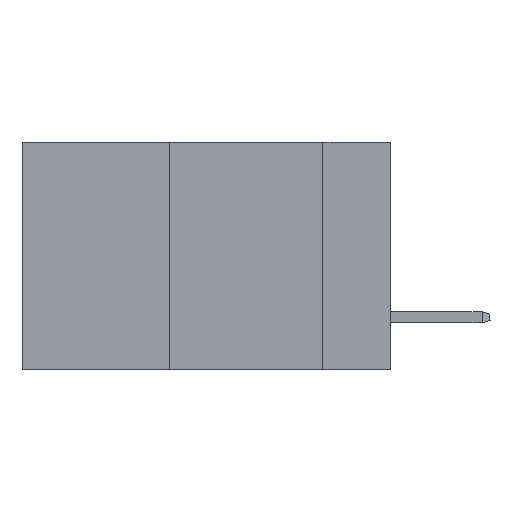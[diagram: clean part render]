
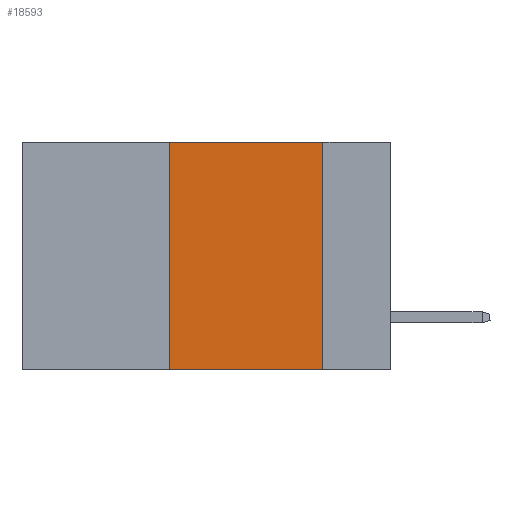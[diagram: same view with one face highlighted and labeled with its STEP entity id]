
A CAD part, left-side view. The second image highlights one B-rep face of the part: STEP entity #18593.
In plain terms, the highlighted planar face has unit normal (-1, 0, 0).
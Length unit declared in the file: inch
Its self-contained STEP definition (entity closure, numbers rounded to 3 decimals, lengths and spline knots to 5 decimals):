
#859 = CARTESIAN_POINT ( 'NONE',  ( 0., 0.11, -0.37 ) ) ;
#862 = CARTESIAN_POINT ( 'NONE',  ( 0., 0.36, 0. ) ) ;
#1056 = DIRECTION ( 'NONE',  ( 0., 0., 1. ) ) ;
#1254 = DIRECTION ( 'NONE',  ( 0., 0., -1. ) ) ;
#1319 = DIRECTION ( 'NONE',  ( 1., 0., 0. ) ) ;
#1737 = VECTOR ( 'NONE', #16440, 39.37008 ) ;
#1964 = ORIENTED_EDGE ( 'NONE', *, *, #2080, .F. ) ;
#2080 = EDGE_CURVE ( 'NONE', #9829, #5342, #14048, .T. ) ;
#2199 = CARTESIAN_POINT ( 'NONE',  ( 0., 0.36, -0.37 ) ) ;
#2877 = PLANE ( 'NONE',  #5099 ) ;
#3153 = VERTEX_POINT ( 'NONE', #859 ) ;
#3887 = LINE ( 'NONE', #7358, #1737 ) ;
#4326 = VERTEX_POINT ( 'NONE', #2199 ) ;
#4347 = CARTESIAN_POINT ( 'NONE',  ( 0., 0.11, 0. ) ) ;
#5099 = AXIS2_PLACEMENT_3D ( 'NONE', #8757, #1319, #1254 ) ;
#5342 = VERTEX_POINT ( 'NONE', #4347 ) ;
#5566 = EDGE_LOOP ( 'NONE', ( #11028, #1964, #9701, #9909 ) ) ;
#6669 = VECTOR ( 'NONE', #1056, 39.37008 ) ;
#7358 = CARTESIAN_POINT ( 'NONE',  ( 0., 0.6, -0.37 ) ) ;
#7507 = FACE_OUTER_BOUND ( 'NONE', #5566, .T. ) ;
#7860 = EDGE_CURVE ( 'NONE', #4326, #9829, #15578, .T. ) ;
#8757 = CARTESIAN_POINT ( 'NONE',  ( 0., 0.6, 0. ) ) ;
#8834 = VECTOR ( 'NONE', #13180, 39.37008 ) ;
#9701 = ORIENTED_EDGE ( 'NONE', *, *, #7860, .F. ) ;
#9829 = VERTEX_POINT ( 'NONE', #15761 ) ;
#9909 = ORIENTED_EDGE ( 'NONE', *, *, #16830, .T. ) ;
#10369 = DIRECTION ( 'NONE',  ( 0., 0., -1. ) ) ;
#11028 = ORIENTED_EDGE ( 'NONE', *, *, #11609, .F. ) ;
#11609 = EDGE_CURVE ( 'NONE', #5342, #3153, #17215, .T. ) ;
#13180 = DIRECTION ( 'NONE',  ( 0., -1., 0. ) ) ;
#14048 = LINE ( 'NONE', #19174, #8834 ) ;
#15578 = LINE ( 'NONE', #862, #6669 ) ;
#15761 = CARTESIAN_POINT ( 'NONE',  ( 0., 0.36, 0. ) ) ;
#16440 = DIRECTION ( 'NONE',  ( 0., -1., 0. ) ) ;
#16830 = EDGE_CURVE ( 'NONE', #4326, #3153, #3887, .T. ) ;
#17215 = LINE ( 'NONE', #19208, #19325 ) ;
#18593 = ADVANCED_FACE ( 'NONE', ( #7507 ), #2877, .F. ) ;
#19174 = CARTESIAN_POINT ( 'NONE',  ( 0., 0.6, 0. ) ) ;
#19208 = CARTESIAN_POINT ( 'NONE',  ( 0., 0.11, 0. ) ) ;
#19325 = VECTOR ( 'NONE', #10369, 39.37008 ) ;
